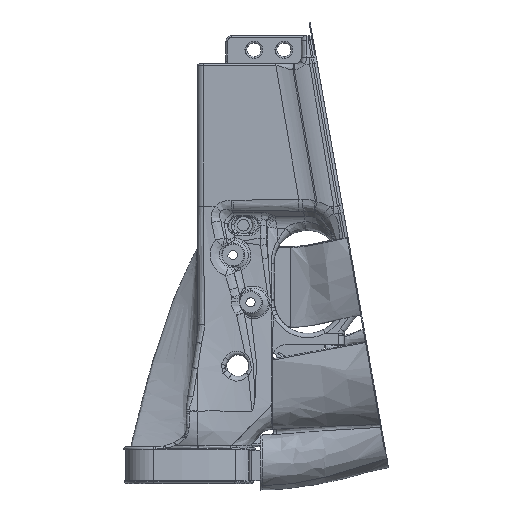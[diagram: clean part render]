
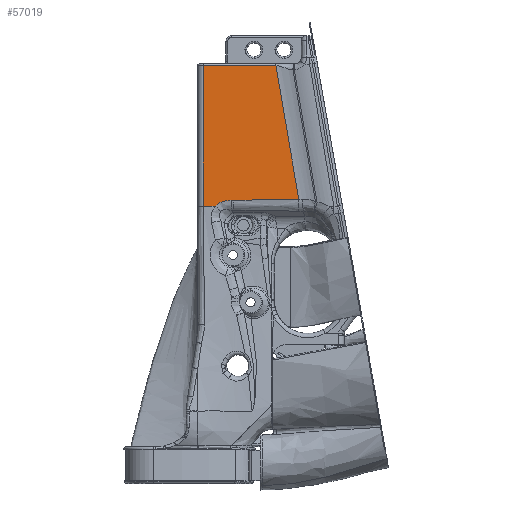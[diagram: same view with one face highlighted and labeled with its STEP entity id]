
A CAD part, left-side view. The second image highlights one B-rep face of the part: STEP entity #57019.
In plain terms, the highlighted planar face has unit normal (-1, 0, 0).
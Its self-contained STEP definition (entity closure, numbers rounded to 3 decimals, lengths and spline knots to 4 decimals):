
#280 = CARTESIAN_POINT ( 'NONE',  ( -0.7, -0.1, 5.29 ) ) ;
#792 = CARTESIAN_POINT ( 'NONE',  ( -0.7, -0.3202, 3.6395 ) ) ;
#2166 = B_SPLINE_CURVE_WITH_KNOTS ( 'NONE', 3,
 ( #50298, #109822, #69697, #28269 ),
 .UNSPECIFIED., .F., .F.,
 ( 4, 4 ),
 ( 0.0279, 0.0571 ),
 .UNSPECIFIED. ) ;
#7071 = EDGE_CURVE ( 'NONE', #120789, #79773, #82295, .T. ) ;
#7864 = LINE ( 'NONE', #59383, #96294 ) ;
#10129 = CARTESIAN_POINT ( 'NONE',  ( -0.7, -0.416, 3.7029 ) ) ;
#12526 = CARTESIAN_POINT ( 'NONE',  ( -0.7, -2.8877, 6.15 ) ) ;
#13848 = VERTEX_POINT ( 'NONE', #126847 ) ;
#14524 = B_SPLINE_CURVE_WITH_KNOTS ( 'NONE', 3,
 ( #73156, #280, #111982, #101941 ),
 .UNSPECIFIED., .F., .F.,
 ( 4, 4 ),
 ( -0.1525, -0.0893 ),
 .UNSPECIFIED. ) ;
#14964 = EDGE_CURVE ( 'NONE', #67746, #13848, #36450, .T. ) ;
#15288 = B_SPLINE_CURVE_WITH_KNOTS ( 'NONE', 3,
 ( #54740, #53422, #116259, #24634 ),
 .UNSPECIFIED., .F., .F.,
 ( 4, 4 ),
 ( 0.5133, 0.64 ),
 .UNSPECIFIED. ) ;
#20853 = CARTESIAN_POINT ( 'NONE',  ( -0.7, -0.5659, 3.7336 ) ) ;
#24220 = CARTESIAN_POINT ( 'NONE',  ( -0.7, -0.2304, 3.63 ) ) ;
#24634 = CARTESIAN_POINT ( 'NONE',  ( -0.7, -0.2304, 3.63 ) ) ;
#26340 = CARTESIAN_POINT ( 'NONE',  ( -0.7, -0.3116, 3.63 ) ) ;
#28269 = CARTESIAN_POINT ( 'NONE',  ( -0.7, -1.7909, 3.7543 ) ) ;
#31350 = DIRECTION ( 'NONE',  ( -1., 0., 0. ) ) ;
#32722 = EDGE_CURVE ( 'NONE', #79773, #108578, #7864, .T. ) ;
#35565 = DIRECTION ( 'NONE',  ( 0., 1., 0. ) ) ;
#36450 = B_SPLINE_CURVE_WITH_KNOTS ( 'NONE', 3,
 ( #24220, #96378, #74361, #86992 ),
 .UNSPECIFIED., .F., .F.,
 ( 4, 4 ),
 ( 0.64, 0.8438 ),
 .UNSPECIFIED. ) ;
#41498 = VECTOR ( 'NONE', #35565, 39.3701 ) ;
#42254 = VERTEX_POINT ( 'NONE', #46622 ) ;
#43032 = ORIENTED_EDGE ( 'NONE', *, *, #61430, .F. ) ;
#45839 = LINE ( 'NONE', #86588, #54424 ) ;
#46622 = CARTESIAN_POINT ( 'NONE',  ( -0.7, -1.3849, 6.12 ) ) ;
#48623 = CARTESIAN_POINT ( 'NONE',  ( -0.7, -0.2304, 3.63 ) ) ;
#50298 = CARTESIAN_POINT ( 'NONE',  ( -0.7, -0.64, 3.7336 ) ) ;
#50327 = CARTESIAN_POINT ( 'NONE',  ( -0.7, -0.5025, 3.7266 ) ) ;
#50989 = CARTESIAN_POINT ( 'NONE',  ( -0.7, -0.4899, 3.7243 ) ) ;
#53190 = ORIENTED_EDGE ( 'NONE', *, *, #14964, .F. ) ;
#53422 = CARTESIAN_POINT ( 'NONE',  ( -0.7, -0.2845, 3.63 ) ) ;
#54424 = VECTOR ( 'NONE', #127442, 39.3701 ) ;
#54740 = CARTESIAN_POINT ( 'NONE',  ( -0.7, -0.3116, 3.63 ) ) ;
#57019 = ADVANCED_FACE ( 'NONE', ( #92848 ), #102222, .T. ) ;
#57127 = VERTEX_POINT ( 'NONE', #97438 ) ;
#59383 = CARTESIAN_POINT ( 'NONE',  ( -0.7, -2.8877, 3.7336 ) ) ;
#60844 = EDGE_CURVE ( 'NONE', #57127, #42254, #45839, .T. ) ;
#61430 = EDGE_CURVE ( 'NONE', #120789, #67746, #15288, .T. ) ;
#62416 = ORIENTED_EDGE ( 'NONE', *, *, #104401, .T. ) ;
#63149 = ORIENTED_EDGE ( 'NONE', *, *, #32722, .T. ) ;
#67746 = VERTEX_POINT ( 'NONE', #48623 ) ;
#69697 = CARTESIAN_POINT ( 'NONE',  ( -0.7, -1.4073, 3.7543 ) ) ;
#70825 = CARTESIAN_POINT ( 'NONE',  ( -0.7, -0.64, 3.7336 ) ) ;
#71060 = CARTESIAN_POINT ( 'NONE',  ( -0.7, -0.3116, 3.63 ) ) ;
#71460 = EDGE_CURVE ( 'NONE', #42254, #130592, #86342, .T. ) ;
#71706 = CARTESIAN_POINT ( 'NONE',  ( -0.7, -0.5916, 3.7336 ) ) ;
#72335 = CARTESIAN_POINT ( 'NONE',  ( -0.7, -0.3601, 3.6722 ) ) ;
#73156 = CARTESIAN_POINT ( 'NONE',  ( -0.7, -0.1, 6.12 ) ) ;
#73662 = CARTESIAN_POINT ( 'NONE',  ( -0.7, -0.3928, 3.6924 ) ) ;
#74361 = CARTESIAN_POINT ( 'NONE',  ( -0.7, -0.1435, 3.63 ) ) ;
#74556 = EDGE_CURVE ( 'NONE', #108578, #57127, #2166, .T. ) ;
#79773 = VERTEX_POINT ( 'NONE', #86129 ) ;
#82295 = B_SPLINE_CURVE_WITH_KNOTS ( 'NONE', 3,
 ( #71060, #792, #114452, #121884, #72335, #73662, #10129, #113800, #83669, #50989, #50327, #111841, #20853, #71706 ),
 .UNSPECIFIED., .F., .F.,
 ( 4, 2, 2, 2, 2, 2, 4 ),
 ( 0., 0.001, 0.002, 0.0039, 0.0049, 0.0059, 0.0078 ),
 .UNSPECIFIED. ) ;
#83669 = CARTESIAN_POINT ( 'NONE',  ( -0.7, -0.4649, 3.7186 ) ) ;
#86129 = CARTESIAN_POINT ( 'NONE',  ( -0.7, -0.5916, 3.7336 ) ) ;
#86342 = LINE ( 'NONE', #105785, #41498 ) ;
#86588 = CARTESIAN_POINT ( 'NONE',  ( -0.7, -1.4229, 5.8986 ) ) ;
#86992 = CARTESIAN_POINT ( 'NONE',  ( -0.7, -0.1, 3.63 ) ) ;
#92848 = FACE_OUTER_BOUND ( 'NONE', #104614, .T. ) ;
#96294 = VECTOR ( 'NONE', #130974, 39.3701 ) ;
#96378 = CARTESIAN_POINT ( 'NONE',  ( -0.7, -0.1869, 3.63 ) ) ;
#97438 = CARTESIAN_POINT ( 'NONE',  ( -0.7, -1.7909, 3.7543 ) ) ;
#101941 = CARTESIAN_POINT ( 'NONE',  ( -0.7, -0.1, 3.63 ) ) ;
#102222 = PLANE ( 'NONE',  #110730 ) ;
#103557 = DIRECTION ( 'NONE',  ( 0., 0., 1. ) ) ;
#104401 = EDGE_CURVE ( 'NONE', #130592, #13848, #14524, .T. ) ;
#104614 = EDGE_LOOP ( 'NONE', ( #117242, #62416, #53190, #43032, #115113, #63149, #129466, #129487 ) ) ;
#105785 = CARTESIAN_POINT ( 'NONE',  ( -0.7, 0., 6.12 ) ) ;
#108578 = VERTEX_POINT ( 'NONE', #70825 ) ;
#109822 = CARTESIAN_POINT ( 'NONE',  ( -0.7, -1.0236, 3.7336 ) ) ;
#110730 = AXIS2_PLACEMENT_3D ( 'NONE', #12526, #31350, #103557 ) ;
#110860 = CARTESIAN_POINT ( 'NONE',  ( -0.7, -0.1, 6.12 ) ) ;
#111841 = CARTESIAN_POINT ( 'NONE',  ( -0.7, -0.5404, 3.732 ) ) ;
#111982 = CARTESIAN_POINT ( 'NONE',  ( -0.7, -0.1, 4.46 ) ) ;
#113800 = CARTESIAN_POINT ( 'NONE',  ( -0.7, -0.4525, 3.7151 ) ) ;
#114452 = CARTESIAN_POINT ( 'NONE',  ( -0.7, -0.3296, 3.6483 ) ) ;
#115113 = ORIENTED_EDGE ( 'NONE', *, *, #7071, .T. ) ;
#116259 = CARTESIAN_POINT ( 'NONE',  ( -0.7, -0.2574, 3.63 ) ) ;
#117242 = ORIENTED_EDGE ( 'NONE', *, *, #71460, .T. ) ;
#120789 = VERTEX_POINT ( 'NONE', #26340 ) ;
#121884 = CARTESIAN_POINT ( 'NONE',  ( -0.7, -0.3495, 3.6646 ) ) ;
#126847 = CARTESIAN_POINT ( 'NONE',  ( -0.7, -0.1, 3.63 ) ) ;
#127442 = DIRECTION ( 'NONE',  ( 0., 0.169, 0.986 ) ) ;
#129466 = ORIENTED_EDGE ( 'NONE', *, *, #74556, .T. ) ;
#129487 = ORIENTED_EDGE ( 'NONE', *, *, #60844, .T. ) ;
#130592 = VERTEX_POINT ( 'NONE', #110860 ) ;
#130974 = DIRECTION ( 'NONE',  ( 0., -1., 0. ) ) ;
